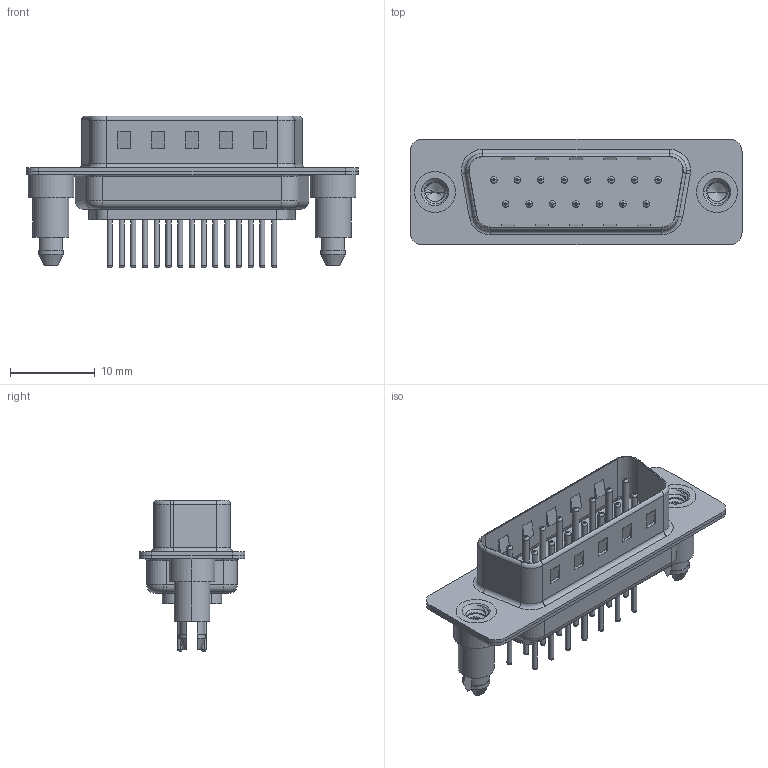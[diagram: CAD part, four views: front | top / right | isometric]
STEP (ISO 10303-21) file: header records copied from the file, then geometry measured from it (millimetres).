
FILE_DESCRIPTION (( 'STEP AP203' ), '1' );
FILE_NAME ('627-M15-320-WN5.STEP', '2020-07-17T00:39:59', ( '' ), ( '' ), 'SwSTEP 2.0', 'SolidWorks 2020', '' );
FILE_SCHEMA (( 'CONFIG_CONTROL_DESIGN' ));
Length unit declared in the file: millimetre
Products named in the file (7): 627M Housing_15 Contacts; 627M Contact Row 1_20; 627M Shell Front_15 Contacts; 627-M15-320-WN5; 627M Contact Row 2_20; 627M Shell Rear_15 Contacts; 627M 4-40 Threaded Boardlock
Assembly tree (20 placements, depth 2):
  627-M15-320-WN5
    627M Housing_15 Contacts
    627M Shell Front_15 Contacts
    627M Shell Rear_15 Contacts
    627M Contact Row 1_20  x8
    627M Contact Row 2_20  x7
    627M 4-40 Threaded Boardlock  x2
Bounding box: 39.2 x 12.5 x 17.9 mm (x, y, z)
Volume: 1977.1 mm3; surface area: 5141.4 mm2
Topology: 20 solids, 20 shells, 945 faces, 2099 edges, 1284 vertices
Faces by surface type: cylinder 375, torus 290, plane 260, cone 14, bspline 6
Entity records: 17778 total; most frequent: CARTESIAN_POINT 4301, DIRECTION 2777, ORIENTED_EDGE 2444, EDGE_CURVE 1222, AXIS2_PLACEMENT_3D 1097, VERTEX_POINT 773, EDGE_LOOP 621, VECTOR 583
